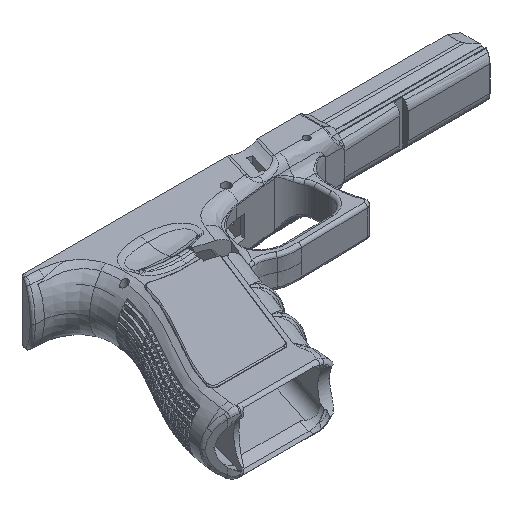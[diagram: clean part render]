
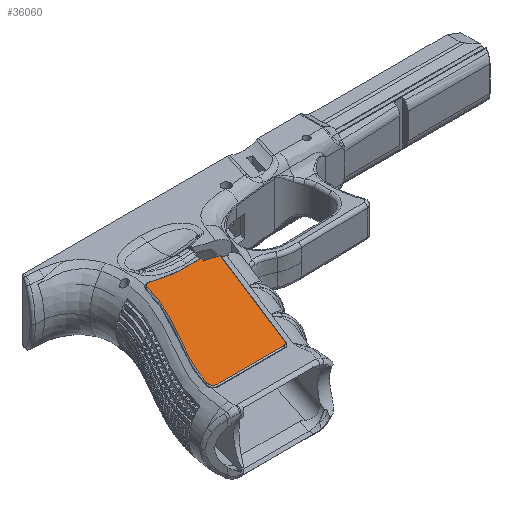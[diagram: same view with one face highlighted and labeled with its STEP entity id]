
A CAD part, isometric view. The second image highlights one B-rep face of the part: STEP entity #36060.
In plain terms, the highlighted planar face has unit normal (0, 0, 1).
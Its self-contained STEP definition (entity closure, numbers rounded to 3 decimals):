
#2474=FACE_OUTER_BOUND('',#4524,.T.);
#4524=EDGE_LOOP('',(#23487,#23488,#23489,#23490,#23491,#23492,#23493,#23494,
#23495,#23496,#23497,#23498));
#6601=B_SPLINE_CURVE_WITH_KNOTS('',3,(#49916,#49917,#49918,#49919,#49920,
#49921,#49922,#49923,#49924,#49925,#49926),.UNSPECIFIED.,.F.,.F.,(4,2,1,
1,1,1,1,4),(-0.017,0.,0.167,0.333,0.5,0.667,
0.833,1.),.UNSPECIFIED.);
#6602=B_SPLINE_CURVE_WITH_KNOTS('',3,(#49930,#49931,#49932,#49933,#49934,
#49935,#49936,#49937,#49938,#49939,#49940,#49941,#49942,#49943,#49944,#49945,
#49946,#49947,#49948),.UNSPECIFIED.,.F.,.F.,(4,1,1,1,1,1,1,1,1,1,1,1,1,
1,1,1,4),(0.,0.04,0.08,0.12,0.16,0.2,0.24,0.28,0.32,0.36,0.4,0.44,0.48,
0.52,0.56,0.6,0.632),.UNSPECIFIED.);
#6603=B_SPLINE_CURVE_WITH_KNOTS('',3,(#49950,#49951,#49952,#49953,#49954,
#49955,#49956),.UNSPECIFIED.,.F.,.F.,(4,1,1,1,4),(0.632,0.64,
0.68,0.72,0.747),.UNSPECIFIED.);
#6604=B_SPLINE_CURVE_WITH_KNOTS('',3,(#49958,#49959,#49960,#49961),
 .UNSPECIFIED.,.F.,.F.,(4,4),(0.747,0.756),
 .UNSPECIFIED.);
#6605=B_SPLINE_CURVE_WITH_KNOTS('',3,(#49963,#49964,#49965,#49966,#49967,
#49968,#49969,#49970,#49971,#49972),.UNSPECIFIED.,.F.,.F.,(4,1,1,1,1,1,
1,4),(0.756,0.76,0.8,0.84,0.88,0.92,0.96,1.),
 .UNSPECIFIED.);
#8103=CIRCLE('',#38134,2.03);
#8104=CIRCLE('',#38135,2.03);
#8105=CIRCLE('',#38136,2.03);
#8757=LINE('',#49906,#11265);
#8758=LINE('',#49910,#11266);
#8759=LINE('',#49912,#11267);
#8760=LINE('',#49914,#11268);
#11265=VECTOR('',#41184,1.015);
#11266=VECTOR('',#41187,1.015);
#11267=VECTOR('',#41188,10.);
#11268=VECTOR('',#41189,10.);
#13784=VERTEX_POINT('',#49904);
#13785=VERTEX_POINT('',#49905);
#13786=VERTEX_POINT('',#49907);
#13787=VERTEX_POINT('',#49909);
#13788=VERTEX_POINT('',#49911);
#13789=VERTEX_POINT('',#49913);
#13790=VERTEX_POINT('',#49915);
#13791=VERTEX_POINT('',#49927);
#13792=VERTEX_POINT('',#49929);
#13793=VERTEX_POINT('',#49949);
#13794=VERTEX_POINT('',#49957);
#13795=VERTEX_POINT('',#49962);
#17610=EDGE_CURVE('',#13784,#13785,#8757,.T.);
#17611=EDGE_CURVE('',#13785,#13786,#8103,.T.);
#17612=EDGE_CURVE('',#13786,#13787,#8758,.T.);
#17613=EDGE_CURVE('',#13787,#13788,#8759,.T.);
#17614=EDGE_CURVE('',#13788,#13789,#8760,.T.);
#17615=EDGE_CURVE('',#13789,#13790,#6601,.T.);
#17616=EDGE_CURVE('',#13790,#13791,#8104,.T.);
#17617=EDGE_CURVE('',#13791,#13792,#6602,.T.);
#17618=EDGE_CURVE('',#13792,#13793,#6603,.T.);
#17619=EDGE_CURVE('',#13793,#13794,#6604,.T.);
#17620=EDGE_CURVE('',#13794,#13795,#6605,.T.);
#17621=EDGE_CURVE('',#13795,#13784,#8105,.T.);
#23487=ORIENTED_EDGE('',*,*,#17610,.T.);
#23488=ORIENTED_EDGE('',*,*,#17611,.T.);
#23489=ORIENTED_EDGE('',*,*,#17612,.T.);
#23490=ORIENTED_EDGE('',*,*,#17613,.T.);
#23491=ORIENTED_EDGE('',*,*,#17614,.T.);
#23492=ORIENTED_EDGE('',*,*,#17615,.T.);
#23493=ORIENTED_EDGE('',*,*,#17616,.T.);
#23494=ORIENTED_EDGE('',*,*,#17617,.T.);
#23495=ORIENTED_EDGE('',*,*,#17618,.T.);
#23496=ORIENTED_EDGE('',*,*,#17619,.T.);
#23497=ORIENTED_EDGE('',*,*,#17620,.T.);
#23498=ORIENTED_EDGE('',*,*,#17621,.T.);
#35229=PLANE('',#38133);
#36060=ADVANCED_FACE('',(#2474),#35229,.T.);
#38133=AXIS2_PLACEMENT_3D('',#49903,#41182,#41183);
#38134=AXIS2_PLACEMENT_3D('',#49908,#41185,#41186);
#38135=AXIS2_PLACEMENT_3D('',#49928,#41190,#41191);
#38136=AXIS2_PLACEMENT_3D('',#49973,#41192,#41193);
#41182=DIRECTION('center_axis',(0.,0.,1.));
#41183=DIRECTION('ref_axis',(1.,0.,0.));
#41184=DIRECTION('',(1.,0.,0.));
#41185=DIRECTION('center_axis',(0.,0.,1.));
#41186=DIRECTION('ref_axis',(0.,-1.,0.));
#41187=DIRECTION('',(0.367,0.93,0.));
#41188=DIRECTION('',(-0.954,0.301,0.));
#41189=DIRECTION('',(0.301,0.954,0.));
#41190=DIRECTION('center_axis',(0.,0.,1.));
#41191=DIRECTION('ref_axis',(0.318,0.948,0.));
#41192=DIRECTION('center_axis',(0.,0.,1.));
#41193=DIRECTION('ref_axis',(-0.96,0.279,0.));
#49903=CARTESIAN_POINT('Origin',(-1.985,0.015,15.194));
#49904=CARTESIAN_POINT('',(-2.094,-92.249,15.194));
#49905=CARTESIAN_POINT('',(29.107,-92.249,15.194));
#49906=CARTESIAN_POINT('',(-2.094,-92.248,15.194));
#49907=CARTESIAN_POINT('',(30.996,-90.962,15.194));
#49908=CARTESIAN_POINT('Origin',(29.107,-90.218,15.194));
#49909=CARTESIAN_POINT('',(50.838,-40.591,15.194));
#49910=CARTESIAN_POINT('',(30.996,-90.962,15.194));
#49911=CARTESIAN_POINT('',(44.842,-38.7,15.194));
#49912=CARTESIAN_POINT('',(17.875,-30.198,15.194));
#49913=CARTESIAN_POINT('',(45.309,-37.219,15.194));
#49914=CARTESIAN_POINT('',(51.169,-18.632,15.194));
#49915=CARTESIAN_POINT('',(23.528,-34.895,15.194));
#49916=CARTESIAN_POINT('Ctrl Pts',(45.309,-37.219,15.194));
#49917=CARTESIAN_POINT('Ctrl Pts',(45.22,-37.224,15.194));
#49918=CARTESIAN_POINT('Ctrl Pts',(45.131,-37.229,15.194));
#49919=CARTESIAN_POINT('Ctrl Pts',(44.149,-37.281,15.194));
#49920=CARTESIAN_POINT('Ctrl Pts',(42.269,-37.356,15.194));
#49921=CARTESIAN_POINT('Ctrl Pts',(39.18,-37.372,15.194));
#49922=CARTESIAN_POINT('Ctrl Pts',(35.79,-37.24,15.194));
#49923=CARTESIAN_POINT('Ctrl Pts',(32.077,-36.885,15.194));
#49924=CARTESIAN_POINT('Ctrl Pts',(28.015,-36.198,15.194));
#49925=CARTESIAN_POINT('Ctrl Pts',(25.055,-35.407,15.194));
#49926=CARTESIAN_POINT('Ctrl Pts',(23.528,-34.895,15.194));
#49927=CARTESIAN_POINT('',(20.911,-36.336,15.194));
#49928=CARTESIAN_POINT('Origin',(22.882,-36.819,15.194));
#49929=CARTESIAN_POINT('',(4.702,-70.389,15.194));
#49930=CARTESIAN_POINT('Ctrl Pts',(20.911,-36.336,15.194));
#49931=CARTESIAN_POINT('Ctrl Pts',(20.827,-36.676,15.194));
#49932=CARTESIAN_POINT('Ctrl Pts',(20.644,-37.398,15.194));
#49933=CARTESIAN_POINT('Ctrl Pts',(20.312,-38.6,15.194));
#49934=CARTESIAN_POINT('Ctrl Pts',(19.914,-39.93,15.194));
#49935=CARTESIAN_POINT('Ctrl Pts',(19.44,-41.391,15.194));
#49936=CARTESIAN_POINT('Ctrl Pts',(18.88,-42.986,15.194));
#49937=CARTESIAN_POINT('Ctrl Pts',(18.224,-44.719,15.194));
#49938=CARTESIAN_POINT('Ctrl Pts',(17.46,-46.593,15.194));
#49939=CARTESIAN_POINT('Ctrl Pts',(16.579,-48.609,15.194));
#49940=CARTESIAN_POINT('Ctrl Pts',(15.572,-50.769,15.194));
#49941=CARTESIAN_POINT('Ctrl Pts',(14.421,-53.098,15.194));
#49942=CARTESIAN_POINT('Ctrl Pts',(13.103,-55.628,15.194));
#49943=CARTESIAN_POINT('Ctrl Pts',(11.599,-58.388,15.194));
#49944=CARTESIAN_POINT('Ctrl Pts',(9.887,-61.417,15.194));
#49945=CARTESIAN_POINT('Ctrl Pts',(7.979,-64.711,15.194));
#49946=CARTESIAN_POINT('Ctrl Pts',(6.175,-67.814,15.194));
#49947=CARTESIAN_POINT('Ctrl Pts',(5.138,-69.622,15.194));
#49948=CARTESIAN_POINT('Ctrl Pts',(4.702,-70.389,15.194));
#49949=CARTESIAN_POINT('',(0.879,-77.452,15.194));
#49950=CARTESIAN_POINT('Ctrl Pts',(4.702,-70.389,15.194));
#49951=CARTESIAN_POINT('Ctrl Pts',(4.592,-70.582,15.194));
#49952=CARTESIAN_POINT('Ctrl Pts',(3.945,-71.723,15.194));
#49953=CARTESIAN_POINT('Ctrl Pts',(2.864,-73.667,15.194));
#49954=CARTESIAN_POINT('Ctrl Pts',(1.739,-75.769,15.194));
#49955=CARTESIAN_POINT('Ctrl Pts',(1.117,-76.98,15.194));
#49956=CARTESIAN_POINT('Ctrl Pts',(0.879,-77.452,
15.194));
#49957=CARTESIAN_POINT('',(0.621,-77.965,15.194));
#49958=CARTESIAN_POINT('Ctrl Pts',(0.879,-77.452,
15.194));
#49959=CARTESIAN_POINT('Ctrl Pts',(0.791,-77.624,
15.194));
#49960=CARTESIAN_POINT('Ctrl Pts',(0.705,-77.795,
15.194));
#49961=CARTESIAN_POINT('Ctrl Pts',(0.621,-77.965,
15.194));
#49962=CARTESIAN_POINT('',(-4.043,-89.651,15.194));
#49963=CARTESIAN_POINT('Ctrl Pts',(0.621,-77.965,
15.194));
#49964=CARTESIAN_POINT('Ctrl Pts',(0.59,-78.027,
15.194));
#49965=CARTESIAN_POINT('Ctrl Pts',(0.214,-78.783,
15.194));
#49966=CARTESIAN_POINT('Ctrl Pts',(-0.457,-80.179,
15.194));
#49967=CARTESIAN_POINT('Ctrl Pts',(-1.282,-82.011,
15.194));
#49968=CARTESIAN_POINT('Ctrl Pts',(-2.067,-83.891,
15.194));
#49969=CARTESIAN_POINT('Ctrl Pts',(-2.791,-85.789,
15.194));
#49970=CARTESIAN_POINT('Ctrl Pts',(-3.453,-87.705,15.194));
#49971=CARTESIAN_POINT('Ctrl Pts',(-3.853,-89.,
15.194));
#49972=CARTESIAN_POINT('Ctrl Pts',(-4.043,-89.651,
15.194));
#49973=CARTESIAN_POINT('Origin',(-2.094,-90.218,15.194));
